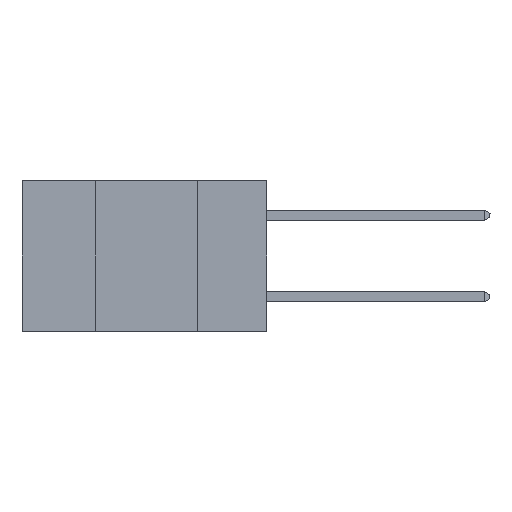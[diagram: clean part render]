
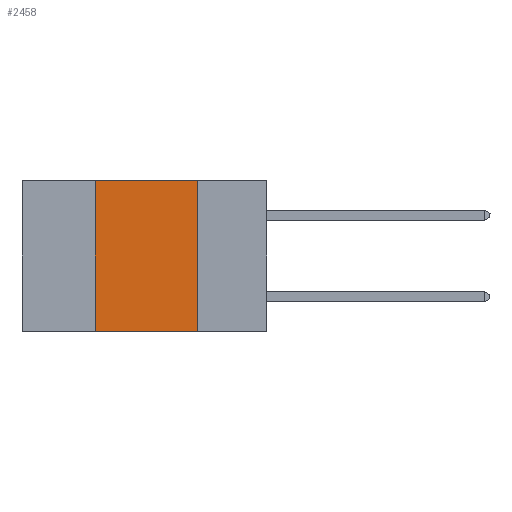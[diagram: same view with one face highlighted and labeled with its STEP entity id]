
A CAD part, left-side view. The second image highlights one B-rep face of the part: STEP entity #2458.
In plain terms, the highlighted planar face has unit normal (-1, 0, 0).
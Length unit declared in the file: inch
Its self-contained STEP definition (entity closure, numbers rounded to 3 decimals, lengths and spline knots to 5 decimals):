
#320 = EDGE_CURVE ( 'NONE', #2783, #10287, #8762, .T. ) ;
#705 = PLANE ( 'NONE',  #8514 ) ;
#751 = EDGE_CURVE ( 'NONE', #14534, #2783, #9073, .T. ) ;
#1086 = CARTESIAN_POINT ( 'NONE',  ( 0., 0.17, -0.37 ) ) ;
#1193 = VERTEX_POINT ( 'NONE', #4657 ) ;
#1531 = ORIENTED_EDGE ( 'NONE', *, *, #13439, .F. ) ;
#1902 = LINE ( 'NONE', #15094, #11377 ) ;
#2078 = DIRECTION ( 'NONE',  ( 0., -1., 0. ) ) ;
#2410 = DIRECTION ( 'NONE',  ( 0., -1., 0. ) ) ;
#2458 = ADVANCED_FACE ( 'NONE', ( #16531 ), #705, .F. ) ;
#2580 = CARTESIAN_POINT ( 'NONE',  ( 0., 0.42, 0. ) ) ;
#2783 = VERTEX_POINT ( 'NONE', #6803 ) ;
#2857 = EDGE_CURVE ( 'NONE', #1193, #10287, #1902, .T. ) ;
#3415 = DIRECTION ( 'NONE',  ( 0., 0., -1. ) ) ;
#3503 = CARTESIAN_POINT ( 'NONE',  ( 0., 0.17, 0. ) ) ;
#4096 = ORIENTED_EDGE ( 'NONE', *, *, #751, .F. ) ;
#4657 = CARTESIAN_POINT ( 'NONE',  ( 0., 0.42, -0.37 ) ) ;
#5098 = ORIENTED_EDGE ( 'NONE', *, *, #320, .F. ) ;
#6342 = CARTESIAN_POINT ( 'NONE',  ( 0., 0.6, 0. ) ) ;
#6803 = CARTESIAN_POINT ( 'NONE',  ( 0., 0.17, 0. ) ) ;
#6839 = VECTOR ( 'NONE', #3415, 39.37008 ) ;
#8514 = AXIS2_PLACEMENT_3D ( 'NONE', #15116, #8753, #13891 ) ;
#8753 = DIRECTION ( 'NONE',  ( 1., 0., 0. ) ) ;
#8762 = LINE ( 'NONE', #3503, #6839 ) ;
#9053 = CARTESIAN_POINT ( 'NONE',  ( 0., 0.42, 0. ) ) ;
#9073 = LINE ( 'NONE', #6342, #14257 ) ;
#10287 = VERTEX_POINT ( 'NONE', #1086 ) ;
#11377 = VECTOR ( 'NONE', #2078, 39.37008 ) ;
#13223 = DIRECTION ( 'NONE',  ( 0., 0., 1. ) ) ;
#13439 = EDGE_CURVE ( 'NONE', #1193, #14534, #14531, .T. ) ;
#13891 = DIRECTION ( 'NONE',  ( 0., 0., -1. ) ) ;
#14257 = VECTOR ( 'NONE', #2410, 39.37008 ) ;
#14531 = LINE ( 'NONE', #2580, #15442 ) ;
#14534 = VERTEX_POINT ( 'NONE', #9053 ) ;
#14611 = ORIENTED_EDGE ( 'NONE', *, *, #2857, .T. ) ;
#15094 = CARTESIAN_POINT ( 'NONE',  ( 0., 0.6, -0.37 ) ) ;
#15116 = CARTESIAN_POINT ( 'NONE',  ( 0., 0.6, 0. ) ) ;
#15442 = VECTOR ( 'NONE', #13223, 39.37008 ) ;
#15684 = EDGE_LOOP ( 'NONE', ( #5098, #4096, #1531, #14611 ) ) ;
#16531 = FACE_OUTER_BOUND ( 'NONE', #15684, .T. ) ;
